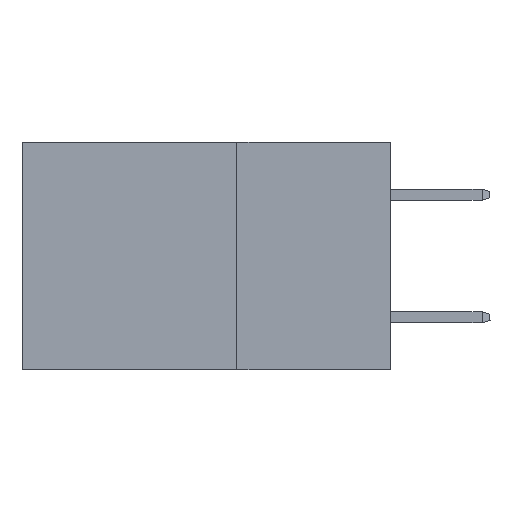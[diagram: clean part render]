
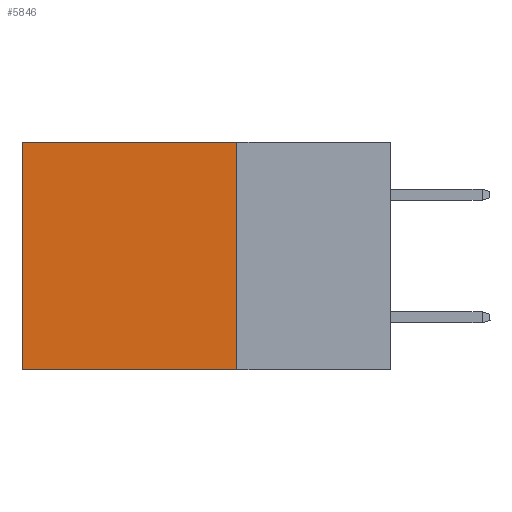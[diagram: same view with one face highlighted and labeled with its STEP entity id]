
A CAD part, left-side view. The second image highlights one B-rep face of the part: STEP entity #5846.
In plain terms, the highlighted planar face has unit normal (-1, 0, 0).
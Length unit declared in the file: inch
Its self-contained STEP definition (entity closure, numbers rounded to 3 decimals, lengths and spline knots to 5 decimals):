
#813 = ORIENTED_EDGE ( 'NONE', *, *, #21648, .F. ) ;
#3735 = EDGE_CURVE ( 'NONE', #15062, #5679, #13194, .T. ) ;
#4069 = CARTESIAN_POINT ( 'NONE',  ( 0.2875, 0.6, -0.37 ) ) ;
#4452 = VECTOR ( 'NONE', #8075, 39.37008 ) ;
#5610 = VECTOR ( 'NONE', #6228, 39.37008 ) ;
#5679 = VERTEX_POINT ( 'NONE', #12725 ) ;
#5846 = ADVANCED_FACE ( 'NONE', ( #10563 ), #5919, .F. ) ;
#5919 = PLANE ( 'NONE',  #15152 ) ;
#6228 = DIRECTION ( 'NONE',  ( 0., 1., 0. ) ) ;
#6477 = CARTESIAN_POINT ( 'NONE',  ( 0.2875, 0.6, 0. ) ) ;
#7229 = LINE ( 'NONE', #6477, #10792 ) ;
#7252 = CARTESIAN_POINT ( 'NONE',  ( 0.2875, 0.25, 0. ) ) ;
#8075 = DIRECTION ( 'NONE',  ( 0., 0., -1. ) ) ;
#8119 = CARTESIAN_POINT ( 'NONE',  ( 0.2875, 0.25, -0.37 ) ) ;
#8548 = VECTOR ( 'NONE', #12465, 39.37008 ) ;
#9328 = ORIENTED_EDGE ( 'NONE', *, *, #21299, .T. ) ;
#9354 = ORIENTED_EDGE ( 'NONE', *, *, #3735, .T. ) ;
#9734 = LINE ( 'NONE', #18479, #4452 ) ;
#9962 = CARTESIAN_POINT ( 'NONE',  ( 0.2875, 0.25, 0. ) ) ;
#10181 = DIRECTION ( 'NONE',  ( 1., 0., 0. ) ) ;
#10563 = FACE_OUTER_BOUND ( 'NONE', #12372, .T. ) ;
#10792 = VECTOR ( 'NONE', #17242, 39.37008 ) ;
#11180 = CARTESIAN_POINT ( 'NONE',  ( 0.2875, 0.25, 0. ) ) ;
#11809 = DIRECTION ( 'NONE',  ( 0., 0., -1. ) ) ;
#12372 = EDGE_LOOP ( 'NONE', ( #9328, #21053, #813, #9354 ) ) ;
#12465 = DIRECTION ( 'NONE',  ( 0., 1., 0. ) ) ;
#12725 = CARTESIAN_POINT ( 'NONE',  ( 0.2875, 0.6, 0. ) ) ;
#13194 = LINE ( 'NONE', #7252, #8548 ) ;
#15062 = VERTEX_POINT ( 'NONE', #11180 ) ;
#15152 = AXIS2_PLACEMENT_3D ( 'NONE', #9962, #10181, #11809 ) ;
#17242 = DIRECTION ( 'NONE',  ( 0., 0., -1. ) ) ;
#17663 = VERTEX_POINT ( 'NONE', #4069 ) ;
#18479 = CARTESIAN_POINT ( 'NONE',  ( 0.2875, 0.25, 0. ) ) ;
#18824 = LINE ( 'NONE', #8119, #5610 ) ;
#19626 = EDGE_CURVE ( 'NONE', #21647, #17663, #18824, .T. ) ;
#19833 = CARTESIAN_POINT ( 'NONE',  ( 0.2875, 0.25, -0.37 ) ) ;
#21053 = ORIENTED_EDGE ( 'NONE', *, *, #19626, .F. ) ;
#21299 = EDGE_CURVE ( 'NONE', #5679, #17663, #7229, .T. ) ;
#21647 = VERTEX_POINT ( 'NONE', #19833 ) ;
#21648 = EDGE_CURVE ( 'NONE', #15062, #21647, #9734, .T. ) ;
